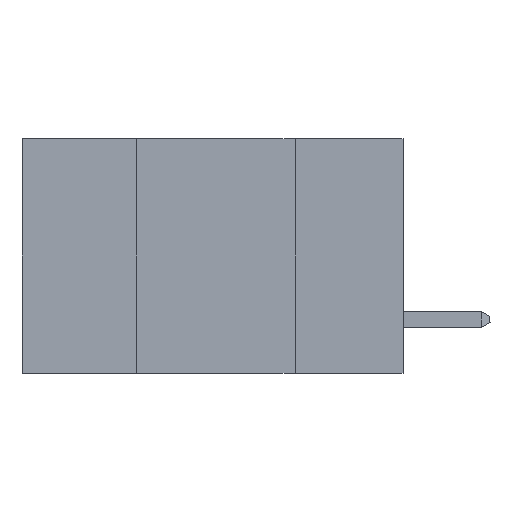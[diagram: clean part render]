
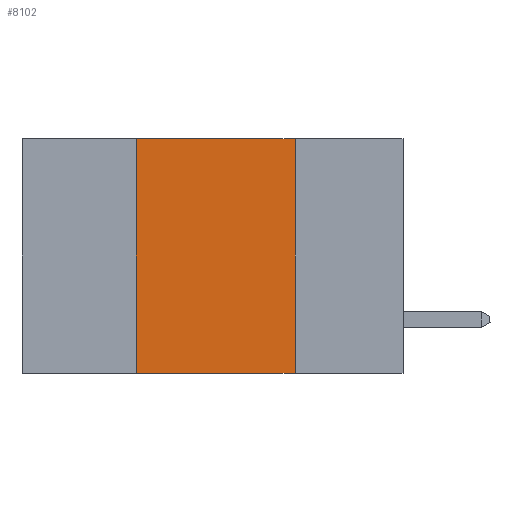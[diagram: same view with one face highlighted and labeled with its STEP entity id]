
A CAD part, left-side view. The second image highlights one B-rep face of the part: STEP entity #8102.
In plain terms, the highlighted planar face has unit normal (-1, 0, 0).
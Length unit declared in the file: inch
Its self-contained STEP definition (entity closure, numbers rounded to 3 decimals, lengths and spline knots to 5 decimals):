
#76 = VECTOR ( 'NONE', #1264, 39.37008 ) ;
#393 = LINE ( 'NONE', #429, #10429 ) ;
#429 = CARTESIAN_POINT ( 'NONE',  ( 0., 0.17, 0. ) ) ;
#890 = EDGE_CURVE ( 'NONE', #12743, #1951, #11777, .T. ) ;
#1264 = DIRECTION ( 'NONE',  ( 0., -1., 0. ) ) ;
#1319 = ORIENTED_EDGE ( 'NONE', *, *, #890, .F. ) ;
#1769 = LINE ( 'NONE', #6810, #76 ) ;
#1951 = VERTEX_POINT ( 'NONE', #13770 ) ;
#3793 = VECTOR ( 'NONE', #3902, 39.37008 ) ;
#3902 = DIRECTION ( 'NONE',  ( 0., -1., 0. ) ) ;
#4502 = EDGE_CURVE ( 'NONE', #1951, #13617, #1769, .T. ) ;
#4762 = VECTOR ( 'NONE', #11753, 39.37008 ) ;
#4780 = LINE ( 'NONE', #5001, #3793 ) ;
#5001 = CARTESIAN_POINT ( 'NONE',  ( 0., 0.6, -0.37 ) ) ;
#5332 = CARTESIAN_POINT ( 'NONE',  ( 0., 0.42, 0. ) ) ;
#5448 = DIRECTION ( 'NONE',  ( 0., 0., -1. ) ) ;
#6086 = DIRECTION ( 'NONE',  ( 1., 0., 0. ) ) ;
#6810 = CARTESIAN_POINT ( 'NONE',  ( 0., 0.6, 0. ) ) ;
#6932 = ORIENTED_EDGE ( 'NONE', *, *, #12454, .T. ) ;
#7956 = DIRECTION ( 'NONE',  ( 0., 0., -1. ) ) ;
#8102 = ADVANCED_FACE ( 'NONE', ( #12699 ), #12285, .F. ) ;
#8283 = CARTESIAN_POINT ( 'NONE',  ( 0., 0.42, -0.37 ) ) ;
#8515 = EDGE_LOOP ( 'NONE', ( #10751, #9037, #1319, #6932 ) ) ;
#8896 = AXIS2_PLACEMENT_3D ( 'NONE', #10304, #6086, #5448 ) ;
#9037 = ORIENTED_EDGE ( 'NONE', *, *, #4502, .F. ) ;
#9979 = CARTESIAN_POINT ( 'NONE',  ( 0., 0.17, -0.37 ) ) ;
#10003 = VERTEX_POINT ( 'NONE', #9979 ) ;
#10304 = CARTESIAN_POINT ( 'NONE',  ( 0., 0.6, 0. ) ) ;
#10429 = VECTOR ( 'NONE', #7956, 39.37008 ) ;
#10712 = CARTESIAN_POINT ( 'NONE',  ( 0., 0.17, 0. ) ) ;
#10751 = ORIENTED_EDGE ( 'NONE', *, *, #13793, .F. ) ;
#11753 = DIRECTION ( 'NONE',  ( 0., 0., 1. ) ) ;
#11777 = LINE ( 'NONE', #5332, #4762 ) ;
#12285 = PLANE ( 'NONE',  #8896 ) ;
#12454 = EDGE_CURVE ( 'NONE', #12743, #10003, #4780, .T. ) ;
#12699 = FACE_OUTER_BOUND ( 'NONE', #8515, .T. ) ;
#12743 = VERTEX_POINT ( 'NONE', #8283 ) ;
#13617 = VERTEX_POINT ( 'NONE', #10712 ) ;
#13770 = CARTESIAN_POINT ( 'NONE',  ( 0., 0.42, 0. ) ) ;
#13793 = EDGE_CURVE ( 'NONE', #13617, #10003, #393, .T. ) ;
